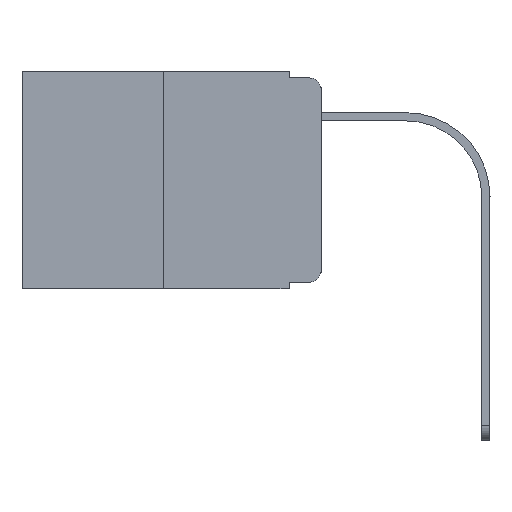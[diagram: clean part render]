
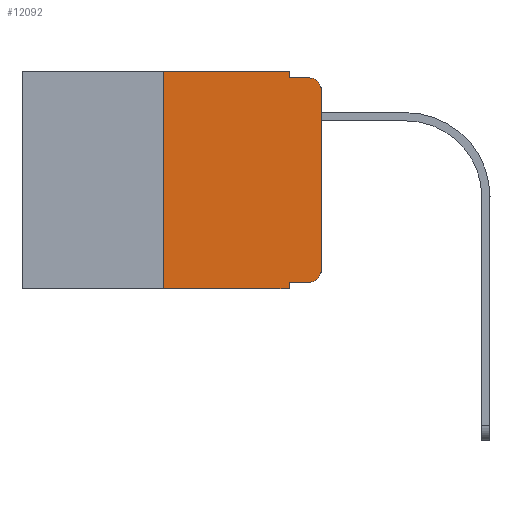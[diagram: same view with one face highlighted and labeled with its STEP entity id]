
A CAD part, left-side view. The second image highlights one B-rep face of the part: STEP entity #12092.
In plain terms, the highlighted planar face has unit normal (-1, 0, 0).
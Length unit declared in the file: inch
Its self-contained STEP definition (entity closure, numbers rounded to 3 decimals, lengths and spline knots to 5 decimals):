
#257 = EDGE_CURVE ( 'NONE', #10197, #5806, #9951, .T. ) ;
#508 = CARTESIAN_POINT ( 'NONE',  ( 0., 0.25, 0. ) ) ;
#1034 = DIRECTION ( 'NONE',  ( 0., 0., -1. ) ) ;
#1462 = VECTOR ( 'NONE', #7085, 39.37008 ) ;
#1655 = VERTEX_POINT ( 'NONE', #15248 ) ;
#1669 = CARTESIAN_POINT ( 'NONE',  ( 0., 0.25, -0.343 ) ) ;
#2728 = CARTESIAN_POINT ( 'NONE',  ( 0., 0.051, -0.01 ) ) ;
#3311 = CARTESIAN_POINT ( 'NONE',  ( 0., 0.051, -0.01 ) ) ;
#3419 = DIRECTION ( 'NONE',  ( 0., -1., 0. ) ) ;
#3543 = EDGE_CURVE ( 'NONE', #4949, #7426, #12568, .T. ) ;
#3793 = DIRECTION ( 'NONE',  ( 0., 0., -1. ) ) ;
#3863 = DIRECTION ( 'NONE',  ( 0., -1., 0. ) ) ;
#4232 = DIRECTION ( 'NONE',  ( 0., 0., -1. ) ) ;
#4426 = DIRECTION ( 'NONE',  ( 0., 0., -1. ) ) ;
#4949 = VERTEX_POINT ( 'NONE', #2728 ) ;
#5158 = CARTESIAN_POINT ( 'NONE',  ( 0., 0.051, 0. ) ) ;
#5185 = ORIENTED_EDGE ( 'NONE', *, *, #16326, .T. ) ;
#5753 = DIRECTION ( 'NONE',  ( -1., 0., 0. ) ) ;
#5806 = VERTEX_POINT ( 'NONE', #15375 ) ;
#5957 = DIRECTION ( 'NONE',  ( 1., 0., 0. ) ) ;
#6031 = ORIENTED_EDGE ( 'NONE', *, *, #14744, .T. ) ;
#6258 = ORIENTED_EDGE ( 'NONE', *, *, #257, .F. ) ;
#6296 = EDGE_CURVE ( 'NONE', #15949, #14981, #12087, .T. ) ;
#6576 = CARTESIAN_POINT ( 'NONE',  ( 0., 0.02, -0.01 ) ) ;
#6846 = VECTOR ( 'NONE', #3419, 39.37008 ) ;
#7085 = DIRECTION ( 'NONE',  ( 0., 0., 1. ) ) ;
#7299 = VECTOR ( 'NONE', #4426, 39.37008 ) ;
#7426 = VERTEX_POINT ( 'NONE', #6576 ) ;
#7651 = CARTESIAN_POINT ( 'NONE',  ( 0., 0.473, 0. ) ) ;
#7711 = ORIENTED_EDGE ( 'NONE', *, *, #3543, .F. ) ;
#8045 = LINE ( 'NONE', #508, #11133 ) ;
#8620 = LINE ( 'NONE', #13467, #1462 ) ;
#9024 = CARTESIAN_POINT ( 'NONE',  ( 0., 0.25, 0. ) ) ;
#9494 = AXIS2_PLACEMENT_3D ( 'NONE', #7651, #5957, #4232 ) ;
#9714 = CARTESIAN_POINT ( 'NONE',  ( 0., 0.02, -0.03 ) ) ;
#9951 = LINE ( 'NONE', #14633, #19192 ) ;
#10197 = VERTEX_POINT ( 'NONE', #9024 ) ;
#10253 = VERTEX_POINT ( 'NONE', #10842 ) ;
#10842 = CARTESIAN_POINT ( 'NONE',  ( 0., 0., -0.03 ) ) ;
#11095 = CARTESIAN_POINT ( 'NONE',  ( 0., 0.051, -0.333 ) ) ;
#11096 = AXIS2_PLACEMENT_3D ( 'NONE', #16593, #5753, #15069 ) ;
#11133 = VECTOR ( 'NONE', #15455, 39.37008 ) ;
#11390 = CIRCLE ( 'NONE', #18207, 0.02 ) ;
#11437 = DIRECTION ( 'NONE',  ( 0., -1., 0. ) ) ;
#12087 = LINE ( 'NONE', #17067, #7299 ) ;
#12092 = ADVANCED_FACE ( 'NONE', ( #15252 ), #16583, .F. ) ;
#12568 = LINE ( 'NONE', #3311, #6846 ) ;
#13058 = LINE ( 'NONE', #17718, #13374 ) ;
#13354 = EDGE_CURVE ( 'NONE', #5806, #4949, #17705, .T. ) ;
#13374 = VECTOR ( 'NONE', #3863, 39.37008 ) ;
#13467 = CARTESIAN_POINT ( 'NONE',  ( 0., 0., 0. ) ) ;
#13590 = EDGE_LOOP ( 'NONE', ( #18036, #18599, #7711, #16327, #6258, #14675, #5185, #15524, #19840, #6031 ) ) ;
#14093 = EDGE_CURVE ( 'NONE', #10253, #7426, #11390, .T. ) ;
#14132 = EDGE_CURVE ( 'NONE', #15949, #18068, #17731, .T. ) ;
#14228 = EDGE_CURVE ( 'NONE', #1655, #10253, #8620, .T. ) ;
#14633 = CARTESIAN_POINT ( 'NONE',  ( 0., 0.473, 0. ) ) ;
#14675 = ORIENTED_EDGE ( 'NONE', *, *, #17024, .F. ) ;
#14744 = EDGE_CURVE ( 'NONE', #18068, #1655, #19529, .T. ) ;
#14981 = VERTEX_POINT ( 'NONE', #15977 ) ;
#15069 = DIRECTION ( 'NONE',  ( 0., 0., -1. ) ) ;
#15248 = CARTESIAN_POINT ( 'NONE',  ( 0., 0., -0.313 ) ) ;
#15252 = FACE_OUTER_BOUND ( 'NONE', #13590, .T. ) ;
#15375 = CARTESIAN_POINT ( 'NONE',  ( 0., 0.051, 0. ) ) ;
#15455 = DIRECTION ( 'NONE',  ( 0., 0., 1. ) ) ;
#15524 = ORIENTED_EDGE ( 'NONE', *, *, #6296, .F. ) ;
#15628 = VECTOR ( 'NONE', #11437, 39.37008 ) ;
#15848 = DIRECTION ( 'NONE',  ( 0., -1., 0. ) ) ;
#15918 = DIRECTION ( 'NONE',  ( -1., 0., 0. ) ) ;
#15949 = VERTEX_POINT ( 'NONE', #11095 ) ;
#15977 = CARTESIAN_POINT ( 'NONE',  ( 0., 0.051, -0.343 ) ) ;
#16326 = EDGE_CURVE ( 'NONE', #17573, #14981, #13058, .T. ) ;
#16327 = ORIENTED_EDGE ( 'NONE', *, *, #13354, .F. ) ;
#16583 = PLANE ( 'NONE',  #9494 ) ;
#16593 = CARTESIAN_POINT ( 'NONE',  ( 0., 0.02, -0.313 ) ) ;
#17024 = EDGE_CURVE ( 'NONE', #17573, #10197, #8045, .T. ) ;
#17067 = CARTESIAN_POINT ( 'NONE',  ( 0., 0.051, 0. ) ) ;
#17222 = VECTOR ( 'NONE', #1034, 39.37008 ) ;
#17573 = VERTEX_POINT ( 'NONE', #1669 ) ;
#17705 = LINE ( 'NONE', #5158, #17222 ) ;
#17718 = CARTESIAN_POINT ( 'NONE',  ( 0., 0.473, -0.343 ) ) ;
#17731 = LINE ( 'NONE', #19641, #15628 ) ;
#18036 = ORIENTED_EDGE ( 'NONE', *, *, #14228, .T. ) ;
#18068 = VERTEX_POINT ( 'NONE', #18910 ) ;
#18207 = AXIS2_PLACEMENT_3D ( 'NONE', #9714, #15918, #3793 ) ;
#18599 = ORIENTED_EDGE ( 'NONE', *, *, #14093, .T. ) ;
#18910 = CARTESIAN_POINT ( 'NONE',  ( 0., 0.02, -0.333 ) ) ;
#19192 = VECTOR ( 'NONE', #15848, 39.37008 ) ;
#19529 = CIRCLE ( 'NONE', #11096, 0.02 ) ;
#19641 = CARTESIAN_POINT ( 'NONE',  ( 0., 0.051, -0.333 ) ) ;
#19840 = ORIENTED_EDGE ( 'NONE', *, *, #14132, .T. ) ;
